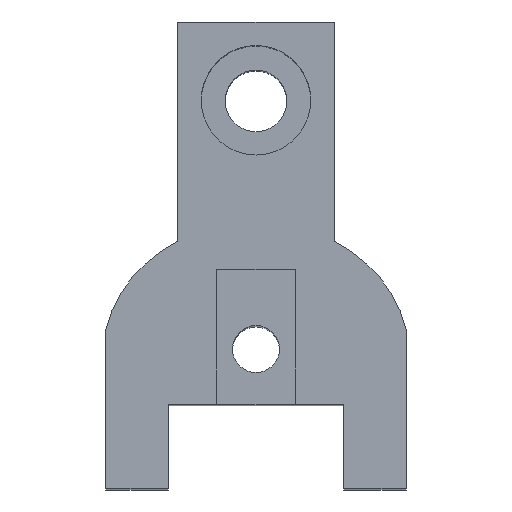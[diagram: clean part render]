
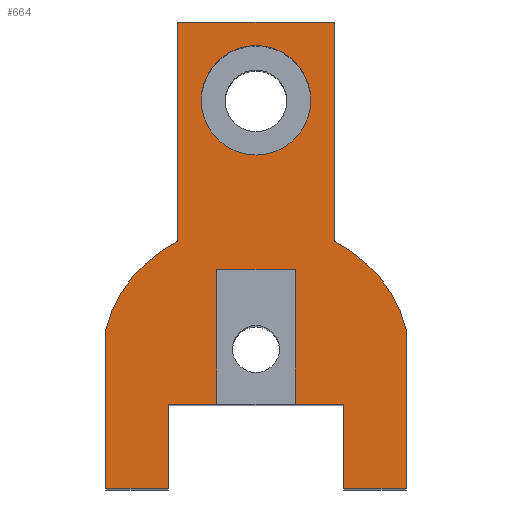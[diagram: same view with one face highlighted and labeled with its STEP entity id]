
A CAD part, top view. The second image highlights one B-rep face of the part: STEP entity #664.
In plain terms, the highlighted planar face has unit normal (0, 0, 1).
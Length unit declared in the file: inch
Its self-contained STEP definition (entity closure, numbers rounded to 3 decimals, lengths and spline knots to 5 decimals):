
#109=CARTESIAN_POINT('',(-0.25,0.36982,3.));
#110=CARTESIAN_POINT('',(-0.30936,0.33892,3.));
#111=CARTESIAN_POINT('',(-0.38203,0.27985,3.));
#112=CARTESIAN_POINT('',(-0.44975,0.17844,3.));
#113=CARTESIAN_POINT('',(-0.47238,0.11901,3.));
#114=CARTESIAN_POINT('',(-0.48,0.08643,3.));
#116=DIRECTION('',(0.,-1.,0.));
#117=VECTOR('',#116,0.70018);
#118=CARTESIAN_POINT('',(-0.25,1.07,3.));
#119=LINE('',#118,#117);
#120=DIRECTION('',(-1.,0.,0.));
#121=VECTOR('',#120,0.5);
#122=CARTESIAN_POINT('',(0.25,1.07,3.));
#123=LINE('',#122,#121);
#124=DIRECTION('',(0.,1.,0.));
#125=VECTOR('',#124,0.70018);
#126=CARTESIAN_POINT('',(0.25,0.36982,3.));
#127=LINE('',#126,#125);
#128=CARTESIAN_POINT('',(0.48,0.08643,3.));
#129=CARTESIAN_POINT('',(0.47238,0.11901,3.));
#130=CARTESIAN_POINT('',(0.44975,0.17844,3.));
#131=CARTESIAN_POINT('',(0.38203,0.27985,3.));
#132=CARTESIAN_POINT('',(0.30936,0.33892,3.));
#133=CARTESIAN_POINT('',(0.25,0.36982,3.));
#135=DIRECTION('',(0.,-1.,0.));
#136=VECTOR('',#135,0.50643);
#137=CARTESIAN_POINT('',(0.48,0.08643,3.));
#138=LINE('',#137,#136);
#139=DIRECTION('',(-1.,0.,0.));
#140=VECTOR('',#139,0.2);
#141=CARTESIAN_POINT('',(0.48,-0.42,3.));
#142=LINE('',#141,#140);
#143=DIRECTION('',(1.,0.,0.));
#144=VECTOR('',#143,0.155);
#145=CARTESIAN_POINT('',(0.125,-0.15132,3.));
#146=LINE('',#145,#144);
#147=DIRECTION('',(0.,1.,0.));
#148=VECTOR('',#147,0.43132);
#149=CARTESIAN_POINT('',(0.125,-0.15132,3.));
#150=LINE('',#149,#148);
#151=DIRECTION('',(-1.,0.,0.));
#152=VECTOR('',#151,0.25);
#153=CARTESIAN_POINT('',(0.125,0.28,3.));
#154=LINE('',#153,#152);
#155=DIRECTION('',(0.,1.,0.));
#156=VECTOR('',#155,0.4313);
#157=CARTESIAN_POINT('',(-0.125,-0.1513,3.));
#158=LINE('',#157,#156);
#159=DIRECTION('',(1.,0.,0.));
#160=VECTOR('',#159,0.155);
#161=CARTESIAN_POINT('',(-0.28,-0.1513,3.));
#162=LINE('',#161,#160);
#163=DIRECTION('',(-1.,0.,0.));
#164=VECTOR('',#163,0.2);
#165=CARTESIAN_POINT('',(-0.28,-0.42,3.));
#166=LINE('',#165,#164);
#167=DIRECTION('',(0.,1.,0.));
#168=VECTOR('',#167,0.50643);
#169=CARTESIAN_POINT('',(-0.48,-0.42,3.));
#170=LINE('',#169,#168);
#171=CARTESIAN_POINT('',(0.,0.82,3.));
#172=DIRECTION('',(0.,0.,1.));
#173=DIRECTION('',(1.,0.,0.));
#174=AXIS2_PLACEMENT_3D('',#171,#172,#173);
#176=CARTESIAN_POINT('',(0.,0.82,3.));
#177=DIRECTION('',(0.,0.,1.));
#178=DIRECTION('',(-1.,0.,0.));
#179=AXIS2_PLACEMENT_3D('',#176,#177,#178);
#235=DIRECTION('',(0.,-1.,0.));
#236=VECTOR('',#235,0.26866);
#237=CARTESIAN_POINT('',(0.28,-0.15134,3.));
#238=LINE('',#237,#236);
#313=DIRECTION('',(0.,1.,0.));
#314=VECTOR('',#313,0.2687);
#315=CARTESIAN_POINT('',(-0.28,-0.42,3.));
#316=LINE('',#315,#314);
#366=CARTESIAN_POINT('',(-0.48,0.08643,3.));
#368=VERTEX_POINT('',#366);
#370=CARTESIAN_POINT('',(0.48,0.08643,3.));
#372=VERTEX_POINT('',#370);
#377=CARTESIAN_POINT('',(0.125,0.28,3.));
#378=CARTESIAN_POINT('',(-0.125,0.28,3.));
#379=VERTEX_POINT('',#377);
#380=VERTEX_POINT('',#378);
#397=CARTESIAN_POINT('',(-0.28,-0.42,3.));
#398=CARTESIAN_POINT('',(-0.48,-0.42,3.));
#399=VERTEX_POINT('',#397);
#400=VERTEX_POINT('',#398);
#401=CARTESIAN_POINT('',(0.48,-0.42,3.));
#402=CARTESIAN_POINT('',(0.28,-0.42,3.));
#403=VERTEX_POINT('',#401);
#404=VERTEX_POINT('',#402);
#406=CARTESIAN_POINT('',(-0.28,-0.1513,3.));
#408=VERTEX_POINT('',#406);
#410=CARTESIAN_POINT('',(0.28,-0.15134,3.));
#412=VERTEX_POINT('',#410);
#413=CARTESIAN_POINT('',(-0.125,-0.1513,3.));
#414=VERTEX_POINT('',#413);
#415=CARTESIAN_POINT('',(0.125,-0.15132,3.));
#416=VERTEX_POINT('',#415);
#455=CARTESIAN_POINT('',(0.25,1.07,3.));
#456=CARTESIAN_POINT('',(-0.25,1.07,3.));
#457=VERTEX_POINT('',#455);
#458=VERTEX_POINT('',#456);
#459=VERTEX_POINT('',#109);
#460=VERTEX_POINT('',#133);
#465=CARTESIAN_POINT('',(0.175,0.82,3.));
#466=CARTESIAN_POINT('',(-0.175,0.82,3.));
#467=VERTEX_POINT('',#465);
#468=VERTEX_POINT('',#466);
#623=CARTESIAN_POINT('',(0.,0.,3.));
#624=DIRECTION('',(0.,0.,1.));
#625=DIRECTION('',(1.,0.,0.));
#626=AXIS2_PLACEMENT_3D('',#623,#624,#625);
#627=PLANE('',#626);
#629=ORIENTED_EDGE('',*,*,#628,.F.);
#631=ORIENTED_EDGE('',*,*,#630,.F.);
#633=ORIENTED_EDGE('',*,*,#632,.F.);
#635=ORIENTED_EDGE('',*,*,#634,.F.);
#637=ORIENTED_EDGE('',*,*,#636,.F.);
#639=ORIENTED_EDGE('',*,*,#638,.T.);
#641=ORIENTED_EDGE('',*,*,#640,.T.);
#643=ORIENTED_EDGE('',*,*,#642,.F.);
#644=ORIENTED_EDGE('',*,*,#581,.F.);
#645=ORIENTED_EDGE('',*,*,#604,.T.);
#646=ORIENTED_EDGE('',*,*,#614,.T.);
#648=ORIENTED_EDGE('',*,*,#647,.F.);
#649=ORIENTED_EDGE('',*,*,#588,.F.);
#651=ORIENTED_EDGE('',*,*,#650,.F.);
#653=ORIENTED_EDGE('',*,*,#652,.T.);
#655=ORIENTED_EDGE('',*,*,#654,.T.);
#656=EDGE_LOOP('',(#629,#631,#633,#635,#637,#639,#641,#643,#644,#645,#646,#648,
#649,#651,#653,#655));
#657=FACE_OUTER_BOUND('',#656,.F.);
#659=ORIENTED_EDGE('',*,*,#658,.T.);
#661=ORIENTED_EDGE('',*,*,#660,.T.);
#662=EDGE_LOOP('',(#659,#661));
#663=FACE_BOUND('',#662,.F.);
#664=ADVANCED_FACE('',(#657,#663),#627,.T.);
#115=B_SPLINE_CURVE_WITH_KNOTS('',3,(#109,#110,#111,#112,#113,#114),
.UNSPECIFIED.,.F.,.F.,(4,1,1,4),(0.,0.5,0.75,1.),.UNSPECIFIED.);
#134=B_SPLINE_CURVE_WITH_KNOTS('',3,(#128,#129,#130,#131,#132,#133),
.UNSPECIFIED.,.F.,.F.,(4,1,1,4),(0.,0.25,0.5,1.),.UNSPECIFIED.);
#175=CIRCLE('',#174,0.175);
#180=CIRCLE('',#179,0.175);
#581=EDGE_CURVE('',#416,#412,#146,.T.);
#588=EDGE_CURVE('',#408,#414,#162,.T.);
#604=EDGE_CURVE('',#416,#379,#150,.T.);
#614=EDGE_CURVE('',#379,#380,#154,.T.);
#628=EDGE_CURVE('',#459,#368,#115,.T.);
#630=EDGE_CURVE('',#458,#459,#119,.T.);
#632=EDGE_CURVE('',#457,#458,#123,.T.);
#634=EDGE_CURVE('',#460,#457,#127,.T.);
#636=EDGE_CURVE('',#372,#460,#134,.T.);
#638=EDGE_CURVE('',#372,#403,#138,.T.);
#640=EDGE_CURVE('',#403,#404,#142,.T.);
#642=EDGE_CURVE('',#412,#404,#238,.T.);
#647=EDGE_CURVE('',#414,#380,#158,.T.);
#650=EDGE_CURVE('',#399,#408,#316,.T.);
#652=EDGE_CURVE('',#399,#400,#166,.T.);
#654=EDGE_CURVE('',#400,#368,#170,.T.);
#658=EDGE_CURVE('',#467,#468,#175,.T.);
#660=EDGE_CURVE('',#468,#467,#180,.T.);
